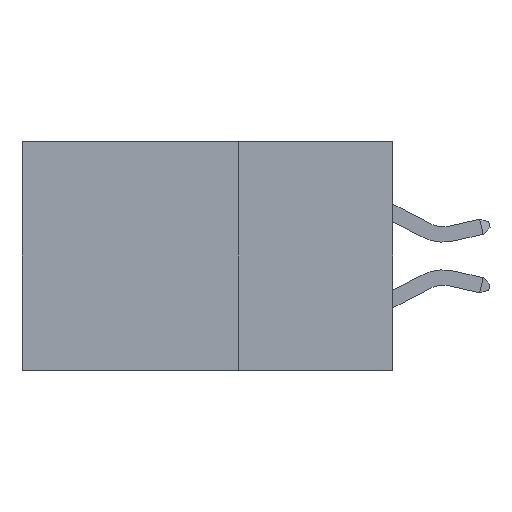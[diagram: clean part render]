
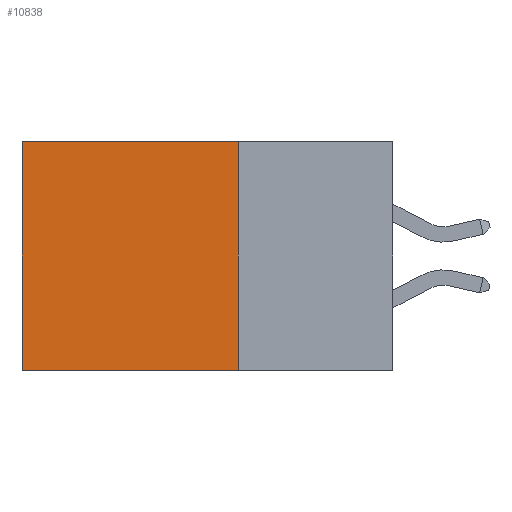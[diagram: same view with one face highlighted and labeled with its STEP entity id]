
A CAD part, left-side view. The second image highlights one B-rep face of the part: STEP entity #10838.
In plain terms, the highlighted planar face has unit normal (-1, 0, 0).
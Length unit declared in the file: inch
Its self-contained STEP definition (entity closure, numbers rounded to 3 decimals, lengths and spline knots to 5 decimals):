
#327 = CARTESIAN_POINT ( 'NONE',  ( 0.2875, 0.6, -0.37 ) ) ;
#833 = CARTESIAN_POINT ( 'NONE',  ( 0.2875, 0.25, -0.37 ) ) ;
#849 = VERTEX_POINT ( 'NONE', #9199 ) ;
#928 = LINE ( 'NONE', #4309, #3867 ) ;
#957 = CARTESIAN_POINT ( 'NONE',  ( 0.2875, 0.25, 0. ) ) ;
#1032 = EDGE_CURVE ( 'NONE', #10066, #8775, #928, .T. ) ;
#1107 = DIRECTION ( 'NONE',  ( 0., 1., 0. ) ) ;
#1306 = ORIENTED_EDGE ( 'NONE', *, *, #3430, .F. ) ;
#1662 = CARTESIAN_POINT ( 'NONE',  ( 0.2875, 0.6, 0. ) ) ;
#2501 = DIRECTION ( 'NONE',  ( 0., 0., -1. ) ) ;
#2855 = DIRECTION ( 'NONE',  ( 0., 0., -1. ) ) ;
#3211 = ORIENTED_EDGE ( 'NONE', *, *, #3695, .T. ) ;
#3269 = FACE_OUTER_BOUND ( 'NONE', #5205, .T. ) ;
#3430 = EDGE_CURVE ( 'NONE', #8775, #4025, #4844, .T. ) ;
#3695 = EDGE_CURVE ( 'NONE', #10066, #849, #4835, .T. ) ;
#3698 = CARTESIAN_POINT ( 'NONE',  ( 0.2875, 0.25, 0. ) ) ;
#3818 = LINE ( 'NONE', #1662, #8576 ) ;
#3867 = VECTOR ( 'NONE', #2501, 39.37008 ) ;
#4025 = VERTEX_POINT ( 'NONE', #327 ) ;
#4309 = CARTESIAN_POINT ( 'NONE',  ( 0.2875, 0.25, 0. ) ) ;
#4559 = DIRECTION ( 'NONE',  ( 1., 0., 0. ) ) ;
#4835 = LINE ( 'NONE', #7012, #5499 ) ;
#4844 = LINE ( 'NONE', #10851, #10783 ) ;
#4990 = DIRECTION ( 'NONE',  ( 0., 1., 0. ) ) ;
#5177 = ORIENTED_EDGE ( 'NONE', *, *, #9476, .T. ) ;
#5205 = EDGE_LOOP ( 'NONE', ( #5177, #1306, #8204, #3211 ) ) ;
#5499 = VECTOR ( 'NONE', #1107, 39.37008 ) ;
#7012 = CARTESIAN_POINT ( 'NONE',  ( 0.2875, 0.25, 0. ) ) ;
#7176 = PLANE ( 'NONE',  #7923 ) ;
#7631 = DIRECTION ( 'NONE',  ( 0., 0., -1. ) ) ;
#7923 = AXIS2_PLACEMENT_3D ( 'NONE', #3698, #4559, #2855 ) ;
#8204 = ORIENTED_EDGE ( 'NONE', *, *, #1032, .F. ) ;
#8576 = VECTOR ( 'NONE', #7631, 39.37008 ) ;
#8775 = VERTEX_POINT ( 'NONE', #833 ) ;
#9199 = CARTESIAN_POINT ( 'NONE',  ( 0.2875, 0.6, 0. ) ) ;
#9476 = EDGE_CURVE ( 'NONE', #849, #4025, #3818, .T. ) ;
#10066 = VERTEX_POINT ( 'NONE', #957 ) ;
#10783 = VECTOR ( 'NONE', #4990, 39.37008 ) ;
#10838 = ADVANCED_FACE ( 'NONE', ( #3269 ), #7176, .F. ) ;
#10851 = CARTESIAN_POINT ( 'NONE',  ( 0.2875, 0.25, -0.37 ) ) ;
